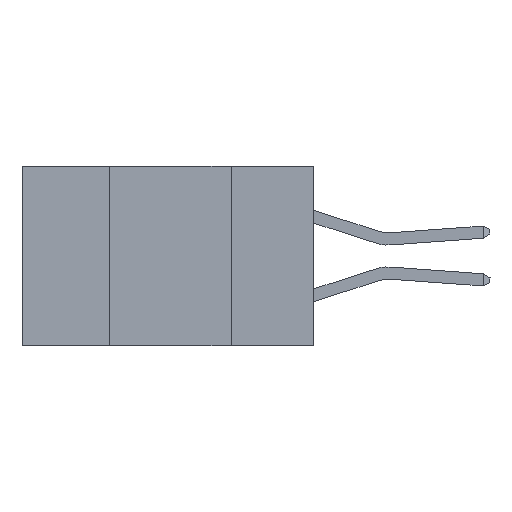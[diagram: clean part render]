
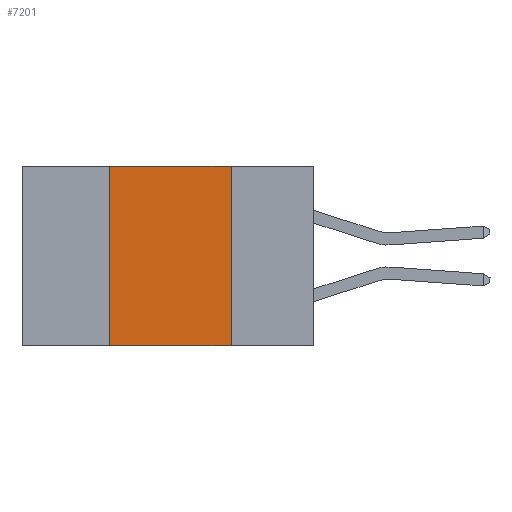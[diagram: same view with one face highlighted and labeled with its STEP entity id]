
A CAD part, left-side view. The second image highlights one B-rep face of the part: STEP entity #7201.
In plain terms, the highlighted planar face has unit normal (-1, 0, 0).
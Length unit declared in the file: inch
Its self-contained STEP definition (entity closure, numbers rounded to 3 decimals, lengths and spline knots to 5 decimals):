
#691 = DIRECTION ( 'NONE',  ( 1., 0., 0. ) ) ;
#980 = CARTESIAN_POINT ( 'NONE',  ( 0., 0.42, 0. ) ) ;
#1070 = CARTESIAN_POINT ( 'NONE',  ( 0., 0.6, -0.37 ) ) ;
#1130 = ORIENTED_EDGE ( 'NONE', *, *, #12835, .F. ) ;
#1232 = LINE ( 'NONE', #1070, #4466 ) ;
#2708 = EDGE_LOOP ( 'NONE', ( #1130, #7739, #4819, #12513 ) ) ;
#2950 = DIRECTION ( 'NONE',  ( 0., 0., 1. ) ) ;
#3174 = CARTESIAN_POINT ( 'NONE',  ( 0., 0.6, 0. ) ) ;
#3558 = DIRECTION ( 'NONE',  ( 0., 0., -1. ) ) ;
#3671 = LINE ( 'NONE', #7292, #9332 ) ;
#3972 = VERTEX_POINT ( 'NONE', #980 ) ;
#4294 = FACE_OUTER_BOUND ( 'NONE', #2708, .T. ) ;
#4298 = VERTEX_POINT ( 'NONE', #11543 ) ;
#4466 = VECTOR ( 'NONE', #12988, 39.37008 ) ;
#4819 = ORIENTED_EDGE ( 'NONE', *, *, #11607, .F. ) ;
#4883 = LINE ( 'NONE', #8224, #6592 ) ;
#5474 = DIRECTION ( 'NONE',  ( 0., 0., -1. ) ) ;
#5777 = EDGE_CURVE ( 'NONE', #3972, #12456, #4883, .T. ) ;
#6379 = CARTESIAN_POINT ( 'NONE',  ( 0., 0.17, 0. ) ) ;
#6592 = VECTOR ( 'NONE', #15475, 39.37008 ) ;
#7201 = ADVANCED_FACE ( 'NONE', ( #4294 ), #8009, .F. ) ;
#7292 = CARTESIAN_POINT ( 'NONE',  ( 0., 0.17, 0. ) ) ;
#7333 = LINE ( 'NONE', #10182, #8444 ) ;
#7739 = ORIENTED_EDGE ( 'NONE', *, *, #5777, .F. ) ;
#7940 = EDGE_CURVE ( 'NONE', #4298, #12615, #1232, .T. ) ;
#8009 = PLANE ( 'NONE',  #13676 ) ;
#8077 = CARTESIAN_POINT ( 'NONE',  ( 0., 0.17, -0.37 ) ) ;
#8224 = CARTESIAN_POINT ( 'NONE',  ( 0., 0.6, 0. ) ) ;
#8444 = VECTOR ( 'NONE', #2950, 39.37008 ) ;
#9332 = VECTOR ( 'NONE', #3558, 39.37008 ) ;
#10182 = CARTESIAN_POINT ( 'NONE',  ( 0., 0.42, 0. ) ) ;
#11543 = CARTESIAN_POINT ( 'NONE',  ( 0., 0.42, -0.37 ) ) ;
#11607 = EDGE_CURVE ( 'NONE', #4298, #3972, #7333, .T. ) ;
#12456 = VERTEX_POINT ( 'NONE', #6379 ) ;
#12513 = ORIENTED_EDGE ( 'NONE', *, *, #7940, .T. ) ;
#12615 = VERTEX_POINT ( 'NONE', #8077 ) ;
#12835 = EDGE_CURVE ( 'NONE', #12456, #12615, #3671, .T. ) ;
#12988 = DIRECTION ( 'NONE',  ( 0., -1., 0. ) ) ;
#13676 = AXIS2_PLACEMENT_3D ( 'NONE', #3174, #691, #5474 ) ;
#15475 = DIRECTION ( 'NONE',  ( 0., -1., 0. ) ) ;
